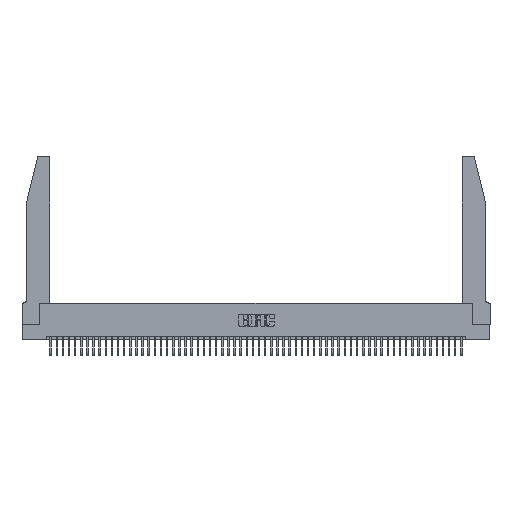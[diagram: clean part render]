
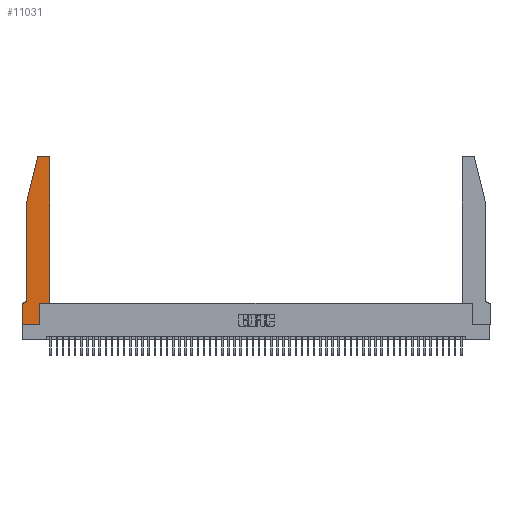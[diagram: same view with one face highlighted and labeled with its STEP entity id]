
A CAD part, top view. The second image highlights one B-rep face of the part: STEP entity #11031.
In plain terms, the highlighted planar face has unit normal (0, 0, 1).
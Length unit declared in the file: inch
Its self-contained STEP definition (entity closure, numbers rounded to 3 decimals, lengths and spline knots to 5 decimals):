
#666 = LINE ( 'NONE', #45448, #30475 ) ;
#937 = VERTEX_POINT ( 'NONE', #21813 ) ;
#1071 = FACE_OUTER_BOUND ( 'NONE', #29831, .T. ) ;
#1600 = VERTEX_POINT ( 'NONE', #26358 ) ;
#2454 = DIRECTION ( 'NONE',  ( 0., -1., 0. ) ) ;
#2721 = EDGE_CURVE ( 'NONE', #24618, #23220, #11589, .T. ) ;
#2906 = ORIENTED_EDGE ( 'NONE', *, *, #15250, .T. ) ;
#3738 = VERTEX_POINT ( 'NONE', #45120 ) ;
#4207 = VECTOR ( 'NONE', #44115, 39.37008 ) ;
#4229 = VERTEX_POINT ( 'NONE', #33361 ) ;
#5478 = AXIS2_PLACEMENT_3D ( 'NONE', #44793, #20549, #48853 ) ;
#6644 = CARTESIAN_POINT ( 'NONE',  ( 0.0755, 0.35, 0.37 ) ) ;
#7001 = AXIS2_PLACEMENT_3D ( 'NONE', #32800, #8592, #36919 ) ;
#8260 = VECTOR ( 'NONE', #26930, 39.37008 ) ;
#8592 = DIRECTION ( 'NONE',  ( 0., 0., -1. ) ) ;
#8825 = CARTESIAN_POINT ( 'NONE',  ( 0.4205, 2.75, 0.37 ) ) ;
#9691 = CARTESIAN_POINT ( 'NONE',  ( 0.4205, 2.72, 0.37 ) ) ;
#10736 = DIRECTION ( 'NONE',  ( 0., 1., 0. ) ) ;
#11031 = ADVANCED_FACE ( 'NONE', ( #1071 ), #14142, .T. ) ;
#11289 = VECTOR ( 'NONE', #17183, 39.37008 ) ;
#11589 = LINE ( 'NONE', #46202, #31839 ) ;
#13174 = CIRCLE ( 'NONE', #7001, 0.07 ) ;
#13761 = DIRECTION ( 'NONE',  ( 1., 0., 0. ) ) ;
#14142 = PLANE ( 'NONE',  #20873 ) ;
#14319 = DIRECTION ( 'NONE',  ( -0.239, -0.971, 0. ) ) ;
#15076 = CARTESIAN_POINT ( 'NONE',  ( 0., 0., 0.37 ) ) ;
#15250 = EDGE_CURVE ( 'NONE', #47886, #44097, #36202, .T. ) ;
#15712 = VECTOR ( 'NONE', #30889, 39.37008 ) ;
#16584 = CIRCLE ( 'NONE', #29641, 0.03 ) ;
#16961 = LINE ( 'NONE', #6644, #15712 ) ;
#17027 = ORIENTED_EDGE ( 'NONE', *, *, #52495, .T. ) ;
#17183 = DIRECTION ( 'NONE',  ( 1., 0., 0. ) ) ;
#17895 = DIRECTION ( 'NONE',  ( 1., 0., 0. ) ) ;
#18175 = CARTESIAN_POINT ( 'NONE',  ( 0.0755, 2., 0.37 ) ) ;
#18584 = VECTOR ( 'NONE', #14319, 39.37008 ) ;
#18846 = LINE ( 'NONE', #30972, #30880 ) ;
#19094 = VERTEX_POINT ( 'NONE', #29434 ) ;
#19137 = VERTEX_POINT ( 'NONE', #29592 ) ;
#20336 = EDGE_CURVE ( 'NONE', #3738, #44502, #16584, .T. ) ;
#20549 = DIRECTION ( 'NONE',  ( 0., 0., 1. ) ) ;
#20873 = AXIS2_PLACEMENT_3D ( 'NONE', #22253, #50572, #26346 ) ;
#21610 = CIRCLE ( 'NONE', #5478, 0.03 ) ;
#21764 = CARTESIAN_POINT ( 'NONE',  ( 0.2865, 0.35, 0.37 ) ) ;
#21813 = CARTESIAN_POINT ( 'NONE',  ( 0.0055, 0.35, 0.37 ) ) ;
#22021 = LINE ( 'NONE', #33256, #11289 ) ;
#22253 = CARTESIAN_POINT ( 'NONE',  ( 0., 0.35, 0.37 ) ) ;
#22461 = CARTESIAN_POINT ( 'NONE',  ( 0., 0., 0.37 ) ) ;
#23036 = EDGE_CURVE ( 'NONE', #28055, #937, #13174, .T. ) ;
#23220 = VERTEX_POINT ( 'NONE', #49786 ) ;
#23739 = EDGE_CURVE ( 'NONE', #937, #47886, #16961, .T. ) ;
#24618 = VERTEX_POINT ( 'NONE', #21764 ) ;
#25276 = DIRECTION ( 'NONE',  ( -1., 0., 0. ) ) ;
#26278 = ORIENTED_EDGE ( 'NONE', *, *, #39048, .T. ) ;
#26346 = DIRECTION ( 'NONE',  ( 1., 0., 0. ) ) ;
#26358 = CARTESIAN_POINT ( 'NONE',  ( 0.2865, 0., 0.37 ) ) ;
#26781 = EDGE_CURVE ( 'NONE', #4229, #19137, #40141, .T. ) ;
#26930 = DIRECTION ( 'NONE',  ( 0., -1., 0. ) ) ;
#26946 = CARTESIAN_POINT ( 'NONE',  ( 0.0755, 0.42, 0.37 ) ) ;
#27501 = VECTOR ( 'NONE', #10736, 39.37008 ) ;
#28055 = VERTEX_POINT ( 'NONE', #26946 ) ;
#28212 = ORIENTED_EDGE ( 'NONE', *, *, #29884, .T. ) ;
#29434 = CARTESIAN_POINT ( 'NONE',  ( 0.284, 2.75, 0.37 ) ) ;
#29592 = CARTESIAN_POINT ( 'NONE',  ( 0.0755, 2., 0.37 ) ) ;
#29641 = AXIS2_PLACEMENT_3D ( 'NONE', #9691, #37995, #13761 ) ;
#29831 = EDGE_LOOP ( 'NONE', ( #26278, #51614, #33878, #28212, #33253, #40916, #2906, #34703, #17027, #42351, #39786, #43585 ) ) ;
#29884 = EDGE_CURVE ( 'NONE', #19137, #28055, #18846, .T. ) ;
#30475 = VECTOR ( 'NONE', #25276, 39.37008 ) ;
#30880 = VECTOR ( 'NONE', #2454, 39.37008 ) ;
#30889 = DIRECTION ( 'NONE',  ( -1., 0., 0. ) ) ;
#30972 = CARTESIAN_POINT ( 'NONE',  ( 0.0755, 2., 0.37 ) ) ;
#31839 = VECTOR ( 'NONE', #17895, 39.37008 ) ;
#32800 = CARTESIAN_POINT ( 'NONE',  ( 0.0055, 0.42, 0.37 ) ) ;
#33253 = ORIENTED_EDGE ( 'NONE', *, *, #23036, .T. ) ;
#33256 = CARTESIAN_POINT ( 'NONE',  ( 0., 0., 0.37 ) ) ;
#33361 = CARTESIAN_POINT ( 'NONE',  ( 0.25487, 2.72718, 0.37 ) ) ;
#33878 = ORIENTED_EDGE ( 'NONE', *, *, #26781, .T. ) ;
#34703 = ORIENTED_EDGE ( 'NONE', *, *, #50256, .T. ) ;
#36202 = LINE ( 'NONE', #15076, #8260 ) ;
#36552 = LINE ( 'NONE', #40074, #4207 ) ;
#36919 = DIRECTION ( 'NONE',  ( -1., 0., 0. ) ) ;
#37995 = DIRECTION ( 'NONE',  ( 0., 0., 1. ) ) ;
#38247 = LINE ( 'NONE', #42951, #27501 ) ;
#38660 = CARTESIAN_POINT ( 'NONE',  ( 0., 0.35, 0.37 ) ) ;
#39048 = EDGE_CURVE ( 'NONE', #44502, #19094, #666, .T. ) ;
#39786 = ORIENTED_EDGE ( 'NONE', *, *, #45436, .T. ) ;
#40074 = CARTESIAN_POINT ( 'NONE',  ( 0.4505, 0.35, 0.37 ) ) ;
#40141 = LINE ( 'NONE', #18175, #18584 ) ;
#40916 = ORIENTED_EDGE ( 'NONE', *, *, #23739, .T. ) ;
#42048 = EDGE_CURVE ( 'NONE', #19094, #4229, #21610, .T. ) ;
#42351 = ORIENTED_EDGE ( 'NONE', *, *, #2721, .T. ) ;
#42951 = CARTESIAN_POINT ( 'NONE',  ( 0.2865, 0.35, 0.37 ) ) ;
#43585 = ORIENTED_EDGE ( 'NONE', *, *, #20336, .T. ) ;
#44097 = VERTEX_POINT ( 'NONE', #22461 ) ;
#44115 = DIRECTION ( 'NONE',  ( 0., 1., 0. ) ) ;
#44502 = VERTEX_POINT ( 'NONE', #8825 ) ;
#44793 = CARTESIAN_POINT ( 'NONE',  ( 0.284, 2.72, 0.37 ) ) ;
#45120 = CARTESIAN_POINT ( 'NONE',  ( 0.4505, 2.72, 0.37 ) ) ;
#45436 = EDGE_CURVE ( 'NONE', #23220, #3738, #36552, .T. ) ;
#45448 = CARTESIAN_POINT ( 'NONE',  ( 0.2605, 2.75, 0.37 ) ) ;
#46202 = CARTESIAN_POINT ( 'NONE',  ( 0.4505, 0.35, 0.37 ) ) ;
#47886 = VERTEX_POINT ( 'NONE', #38660 ) ;
#48853 = DIRECTION ( 'NONE',  ( 1., 0., 0. ) ) ;
#49786 = CARTESIAN_POINT ( 'NONE',  ( 0.4505, 0.35, 0.37 ) ) ;
#50256 = EDGE_CURVE ( 'NONE', #44097, #1600, #22021, .T. ) ;
#50572 = DIRECTION ( 'NONE',  ( 0., 0., 1. ) ) ;
#51614 = ORIENTED_EDGE ( 'NONE', *, *, #42048, .T. ) ;
#52495 = EDGE_CURVE ( 'NONE', #1600, #24618, #38247, .T. ) ;
